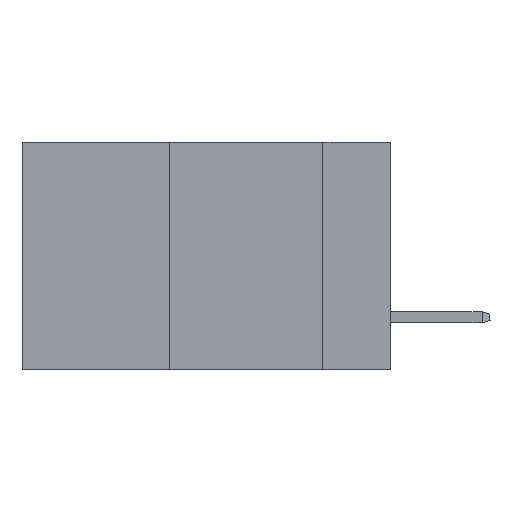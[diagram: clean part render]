
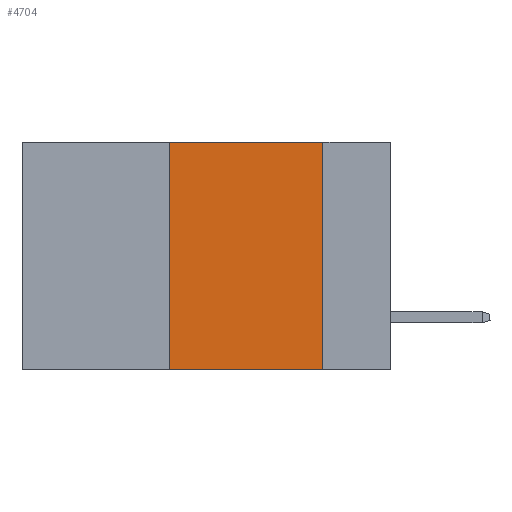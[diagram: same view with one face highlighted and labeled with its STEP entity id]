
A CAD part, left-side view. The second image highlights one B-rep face of the part: STEP entity #4704.
In plain terms, the highlighted planar face has unit normal (-1, 0, 0).
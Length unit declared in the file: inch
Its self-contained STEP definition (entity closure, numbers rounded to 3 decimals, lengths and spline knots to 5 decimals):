
#517 = EDGE_CURVE ( 'NONE', #19753, #18970, #39661, .T. ) ;
#1877 = DIRECTION ( 'NONE',  ( 0., 0., 1. ) ) ;
#2072 = LINE ( 'NONE', #39087, #29956 ) ;
#4105 = DIRECTION ( 'NONE',  ( 0., 0., -1. ) ) ;
#4704 = ADVANCED_FACE ( 'NONE', ( #29276 ), #11886, .F. ) ;
#5034 = CARTESIAN_POINT ( 'NONE',  ( 0., 0.36, -0.37 ) ) ;
#5822 = DIRECTION ( 'NONE',  ( 0., -1., 0. ) ) ;
#9362 = DIRECTION ( 'NONE',  ( 0., 0., -1. ) ) ;
#9519 = ORIENTED_EDGE ( 'NONE', *, *, #9612, .T. ) ;
#9612 = EDGE_CURVE ( 'NONE', #19753, #43492, #44502, .T. ) ;
#11886 = PLANE ( 'NONE',  #21390 ) ;
#12215 = CARTESIAN_POINT ( 'NONE',  ( 0., 0.6, 0. ) ) ;
#16086 = CARTESIAN_POINT ( 'NONE',  ( 0., 0.11, 0. ) ) ;
#16858 = CARTESIAN_POINT ( 'NONE',  ( 0., 0.36, 0. ) ) ;
#17270 = ORIENTED_EDGE ( 'NONE', *, *, #517, .F. ) ;
#18550 = LINE ( 'NONE', #23934, #35687 ) ;
#18970 = VERTEX_POINT ( 'NONE', #37002 ) ;
#19753 = VERTEX_POINT ( 'NONE', #5034 ) ;
#21390 = AXIS2_PLACEMENT_3D ( 'NONE', #12215, #46320, #4105 ) ;
#23934 = CARTESIAN_POINT ( 'NONE',  ( 0., 0.11, 0. ) ) ;
#29276 = FACE_OUTER_BOUND ( 'NONE', #29412, .T. ) ;
#29412 = EDGE_LOOP ( 'NONE', ( #40856, #43762, #17270, #9519 ) ) ;
#29956 = VECTOR ( 'NONE', #47405, 39.37008 ) ;
#31500 = VECTOR ( 'NONE', #5822, 39.37008 ) ;
#33499 = EDGE_CURVE ( 'NONE', #45545, #43492, #18550, .T. ) ;
#35214 = CARTESIAN_POINT ( 'NONE',  ( 0., 0.6, -0.37 ) ) ;
#35687 = VECTOR ( 'NONE', #9362, 39.37008 ) ;
#36656 = VECTOR ( 'NONE', #1877, 39.37008 ) ;
#37002 = CARTESIAN_POINT ( 'NONE',  ( 0., 0.36, 0. ) ) ;
#37428 = EDGE_CURVE ( 'NONE', #18970, #45545, #2072, .T. ) ;
#39087 = CARTESIAN_POINT ( 'NONE',  ( 0., 0.6, 0. ) ) ;
#39661 = LINE ( 'NONE', #16858, #36656 ) ;
#40856 = ORIENTED_EDGE ( 'NONE', *, *, #33499, .F. ) ;
#42332 = CARTESIAN_POINT ( 'NONE',  ( 0., 0.11, -0.37 ) ) ;
#43492 = VERTEX_POINT ( 'NONE', #42332 ) ;
#43762 = ORIENTED_EDGE ( 'NONE', *, *, #37428, .F. ) ;
#44502 = LINE ( 'NONE', #35214, #31500 ) ;
#45545 = VERTEX_POINT ( 'NONE', #16086 ) ;
#46320 = DIRECTION ( 'NONE',  ( 1., 0., 0. ) ) ;
#47405 = DIRECTION ( 'NONE',  ( 0., -1., 0. ) ) ;
